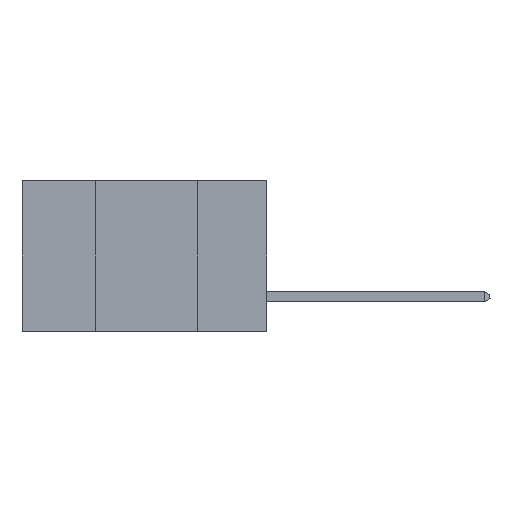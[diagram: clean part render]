
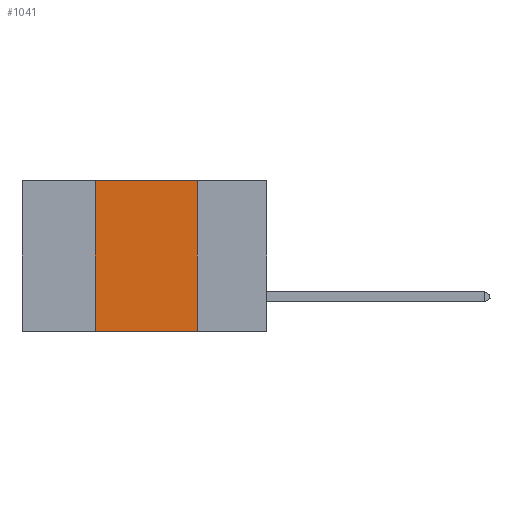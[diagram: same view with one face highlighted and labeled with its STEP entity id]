
A CAD part, left-side view. The second image highlights one B-rep face of the part: STEP entity #1041.
In plain terms, the highlighted planar face has unit normal (-1, 0, 0).
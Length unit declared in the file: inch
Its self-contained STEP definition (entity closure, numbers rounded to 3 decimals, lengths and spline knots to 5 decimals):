
#18 = CARTESIAN_POINT ( 'NONE',  ( 0., 0.6, 0. ) ) ;
#174 = EDGE_CURVE ( 'NONE', #2324, #4411, #13253, .T. ) ;
#370 = CARTESIAN_POINT ( 'NONE',  ( 0., 0.6, 0. ) ) ;
#778 = CARTESIAN_POINT ( 'NONE',  ( 0., 0.17, 0. ) ) ;
#870 = DIRECTION ( 'NONE',  ( 0., 0., -1. ) ) ;
#1041 = ADVANCED_FACE ( 'NONE', ( #11897 ), #1430, .F. ) ;
#1221 = CARTESIAN_POINT ( 'NONE',  ( 0., 0.17, -0.37 ) ) ;
#1430 = PLANE ( 'NONE',  #3363 ) ;
#2130 = EDGE_LOOP ( 'NONE', ( #12635, #11547, #6362, #13526 ) ) ;
#2141 = CARTESIAN_POINT ( 'NONE',  ( 0., 0.42, 0. ) ) ;
#2324 = VERTEX_POINT ( 'NONE', #13934 ) ;
#2508 = CARTESIAN_POINT ( 'NONE',  ( 0., 0.6, -0.37 ) ) ;
#2742 = VECTOR ( 'NONE', #9640, 39.37008 ) ;
#2799 = DIRECTION ( 'NONE',  ( 1., 0., 0. ) ) ;
#3251 = LINE ( 'NONE', #6229, #5948 ) ;
#3363 = AXIS2_PLACEMENT_3D ( 'NONE', #370, #2799, #4027 ) ;
#3841 = VECTOR ( 'NONE', #870, 39.37008 ) ;
#4027 = DIRECTION ( 'NONE',  ( 0., 0., -1. ) ) ;
#4411 = VERTEX_POINT ( 'NONE', #1221 ) ;
#4764 = DIRECTION ( 'NONE',  ( 0., -1., 0. ) ) ;
#5412 = EDGE_CURVE ( 'NONE', #2324, #15387, #3251, .T. ) ;
#5948 = VECTOR ( 'NONE', #14856, 39.37008 ) ;
#5996 = LINE ( 'NONE', #18, #2742 ) ;
#6229 = CARTESIAN_POINT ( 'NONE',  ( 0., 0.42, 0. ) ) ;
#6362 = ORIENTED_EDGE ( 'NONE', *, *, #5412, .F. ) ;
#7587 = VECTOR ( 'NONE', #4764, 39.37008 ) ;
#8666 = EDGE_CURVE ( 'NONE', #9980, #4411, #15394, .T. ) ;
#9640 = DIRECTION ( 'NONE',  ( 0., -1., 0. ) ) ;
#9980 = VERTEX_POINT ( 'NONE', #14700 ) ;
#11547 = ORIENTED_EDGE ( 'NONE', *, *, #12989, .F. ) ;
#11897 = FACE_OUTER_BOUND ( 'NONE', #2130, .T. ) ;
#12635 = ORIENTED_EDGE ( 'NONE', *, *, #8666, .F. ) ;
#12989 = EDGE_CURVE ( 'NONE', #15387, #9980, #5996, .T. ) ;
#13253 = LINE ( 'NONE', #2508, #7587 ) ;
#13526 = ORIENTED_EDGE ( 'NONE', *, *, #174, .T. ) ;
#13934 = CARTESIAN_POINT ( 'NONE',  ( 0., 0.42, -0.37 ) ) ;
#14700 = CARTESIAN_POINT ( 'NONE',  ( 0., 0.17, 0. ) ) ;
#14856 = DIRECTION ( 'NONE',  ( 0., 0., 1. ) ) ;
#15387 = VERTEX_POINT ( 'NONE', #2141 ) ;
#15394 = LINE ( 'NONE', #778, #3841 ) ;
